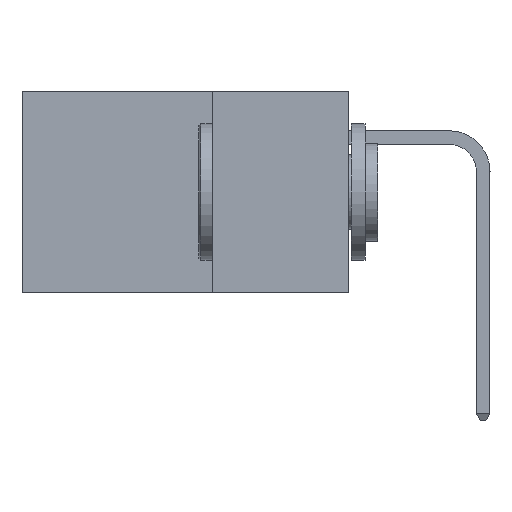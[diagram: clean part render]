
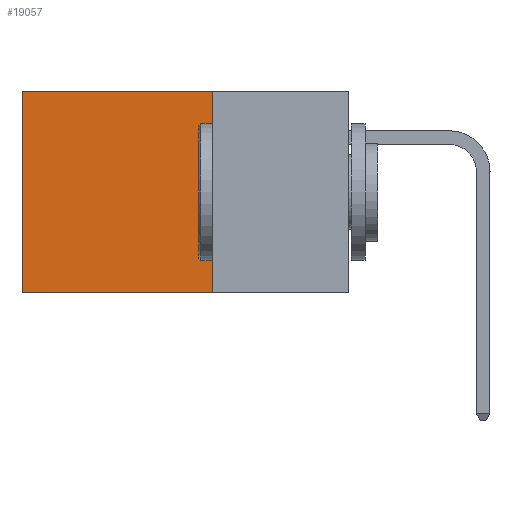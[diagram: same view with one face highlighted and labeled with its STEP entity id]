
A CAD part, left-side view. The second image highlights one B-rep face of the part: STEP entity #19057.
In plain terms, the highlighted planar face has unit normal (-1, 0, 0).
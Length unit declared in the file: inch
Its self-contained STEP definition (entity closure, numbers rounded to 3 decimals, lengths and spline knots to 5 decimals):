
#383 = EDGE_CURVE ( 'NONE', #22483, #17296, #17638, .T. ) ;
#601 = CARTESIAN_POINT ( 'NONE',  ( 0.2875, 0.6, 0. ) ) ;
#1213 = ORIENTED_EDGE ( 'NONE', *, *, #383, .F. ) ;
#1760 = CARTESIAN_POINT ( 'NONE',  ( 0.2875, 0.25, 0. ) ) ;
#3393 = DIRECTION ( 'NONE',  ( 0., 0., -1. ) ) ;
#4735 = EDGE_CURVE ( 'NONE', #22997, #32620, #9978, .T. ) ;
#5063 = EDGE_CURVE ( 'NONE', #32620, #17296, #21232, .T. ) ;
#6207 = PLANE ( 'NONE',  #20159 ) ;
#7679 = CARTESIAN_POINT ( 'NONE',  ( 0.2875, 0.25, 0. ) ) ;
#7952 = CARTESIAN_POINT ( 'NONE',  ( 0.2875, 0.6, -0.37 ) ) ;
#8990 = VECTOR ( 'NONE', #32477, 39.37008 ) ;
#9141 = DIRECTION ( 'NONE',  ( 1., 0., 0. ) ) ;
#9978 = LINE ( 'NONE', #7679, #31841 ) ;
#10451 = EDGE_CURVE ( 'NONE', #22997, #22483, #24707, .T. ) ;
#12713 = EDGE_LOOP ( 'NONE', ( #28379, #1213, #28966, #28025 ) ) ;
#16132 = FACE_OUTER_BOUND ( 'NONE', #12713, .T. ) ;
#16193 = DIRECTION ( 'NONE',  ( 0., 0., -1. ) ) ;
#16244 = VECTOR ( 'NONE', #16193, 39.37008 ) ;
#17296 = VERTEX_POINT ( 'NONE', #7952 ) ;
#17638 = LINE ( 'NONE', #18374, #8990 ) ;
#18374 = CARTESIAN_POINT ( 'NONE',  ( 0.2875, 0.25, -0.37 ) ) ;
#19057 = ADVANCED_FACE ( 'NONE', ( #16132 ), #6207, .F. ) ;
#20013 = CARTESIAN_POINT ( 'NONE',  ( 0.2875, 0.25, -0.37 ) ) ;
#20159 = AXIS2_PLACEMENT_3D ( 'NONE', #26343, #9141, #29189 ) ;
#21232 = LINE ( 'NONE', #26012, #22130 ) ;
#22130 = VECTOR ( 'NONE', #3393, 39.37008 ) ;
#22483 = VERTEX_POINT ( 'NONE', #20013 ) ;
#22997 = VERTEX_POINT ( 'NONE', #27805 ) ;
#24707 = LINE ( 'NONE', #1760, #16244 ) ;
#24932 = DIRECTION ( 'NONE',  ( 0., 1., 0. ) ) ;
#26012 = CARTESIAN_POINT ( 'NONE',  ( 0.2875, 0.6, 0. ) ) ;
#26343 = CARTESIAN_POINT ( 'NONE',  ( 0.2875, 0.25, 0. ) ) ;
#27805 = CARTESIAN_POINT ( 'NONE',  ( 0.2875, 0.25, 0. ) ) ;
#28025 = ORIENTED_EDGE ( 'NONE', *, *, #4735, .T. ) ;
#28379 = ORIENTED_EDGE ( 'NONE', *, *, #5063, .T. ) ;
#28966 = ORIENTED_EDGE ( 'NONE', *, *, #10451, .F. ) ;
#29189 = DIRECTION ( 'NONE',  ( 0., 0., -1. ) ) ;
#31841 = VECTOR ( 'NONE', #24932, 39.37008 ) ;
#32477 = DIRECTION ( 'NONE',  ( 0., 1., 0. ) ) ;
#32620 = VERTEX_POINT ( 'NONE', #601 ) ;
